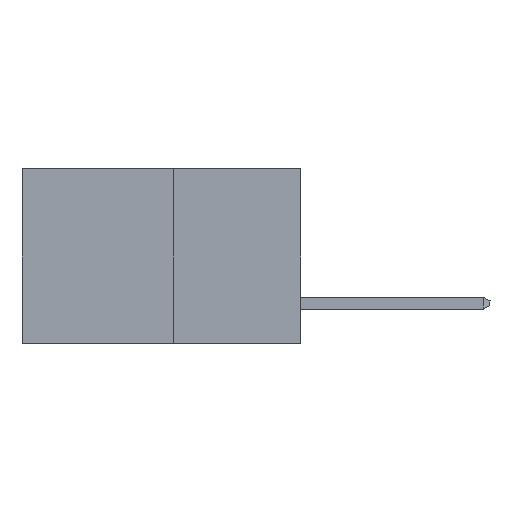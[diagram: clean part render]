
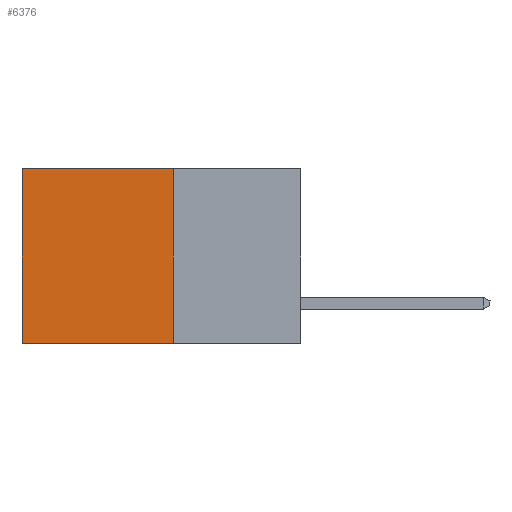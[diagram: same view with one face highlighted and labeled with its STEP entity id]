
A CAD part, left-side view. The second image highlights one B-rep face of the part: STEP entity #6376.
In plain terms, the highlighted planar face has unit normal (-1, 0, 0).
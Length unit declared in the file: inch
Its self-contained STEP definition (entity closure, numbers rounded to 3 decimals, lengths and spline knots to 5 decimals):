
#24 = EDGE_CURVE ( 'NONE', #12196, #17083, #17181, .T. ) ;
#222 = VERTEX_POINT ( 'NONE', #9934 ) ;
#316 = LINE ( 'NONE', #12168, #14150 ) ;
#854 = CARTESIAN_POINT ( 'NONE',  ( 0.277, 0.59, 0. ) ) ;
#1708 = EDGE_LOOP ( 'NONE', ( #17193, #6873, #13920, #2219 ) ) ;
#2219 = ORIENTED_EDGE ( 'NONE', *, *, #24, .T. ) ;
#3734 = DIRECTION ( 'NONE',  ( 1., 0., 0. ) ) ;
#3735 = AXIS2_PLACEMENT_3D ( 'NONE', #12021, #3734, #13391 ) ;
#4505 = VERTEX_POINT ( 'NONE', #7447 ) ;
#5271 = VECTOR ( 'NONE', #15471, 39.37008 ) ;
#5319 = DIRECTION ( 'NONE',  ( 0., 0., -1. ) ) ;
#5929 = CARTESIAN_POINT ( 'NONE',  ( 0.277, 0.27, -0.37 ) ) ;
#6088 = EDGE_CURVE ( 'NONE', #12196, #4505, #12887, .T. ) ;
#6343 = CARTESIAN_POINT ( 'NONE',  ( 0.277, 0.27, 0. ) ) ;
#6376 = ADVANCED_FACE ( 'NONE', ( #12042 ), #6541, .F. ) ;
#6541 = PLANE ( 'NONE',  #3735 ) ;
#6873 = ORIENTED_EDGE ( 'NONE', *, *, #12898, .F. ) ;
#7422 = CARTESIAN_POINT ( 'NONE',  ( 0.277, 0.27, -0.37 ) ) ;
#7447 = CARTESIAN_POINT ( 'NONE',  ( 0.277, 0.27, -0.37 ) ) ;
#9418 = LINE ( 'NONE', #5929, #5271 ) ;
#9934 = CARTESIAN_POINT ( 'NONE',  ( 0.277, 0.59, -0.37 ) ) ;
#10205 = VECTOR ( 'NONE', #12155, 39.37008 ) ;
#10402 = EDGE_CURVE ( 'NONE', #17083, #222, #316, .T. ) ;
#12021 = CARTESIAN_POINT ( 'NONE',  ( 0.277, 0.27, -0.37 ) ) ;
#12042 = FACE_OUTER_BOUND ( 'NONE', #1708, .T. ) ;
#12155 = DIRECTION ( 'NONE',  ( 0., 1., 0. ) ) ;
#12168 = CARTESIAN_POINT ( 'NONE',  ( 0.277, 0.59, -0.37 ) ) ;
#12196 = VERTEX_POINT ( 'NONE', #14121 ) ;
#12887 = LINE ( 'NONE', #7422, #16733 ) ;
#12898 = EDGE_CURVE ( 'NONE', #4505, #222, #9418, .T. ) ;
#13391 = DIRECTION ( 'NONE',  ( 0., 0., -1. ) ) ;
#13920 = ORIENTED_EDGE ( 'NONE', *, *, #6088, .F. ) ;
#14121 = CARTESIAN_POINT ( 'NONE',  ( 0.277, 0.27, 0. ) ) ;
#14150 = VECTOR ( 'NONE', #5319, 39.37008 ) ;
#15471 = DIRECTION ( 'NONE',  ( 0., 1., 0. ) ) ;
#16725 = DIRECTION ( 'NONE',  ( 0., 0., -1. ) ) ;
#16733 = VECTOR ( 'NONE', #16725, 39.37008 ) ;
#17083 = VERTEX_POINT ( 'NONE', #854 ) ;
#17181 = LINE ( 'NONE', #6343, #10205 ) ;
#17193 = ORIENTED_EDGE ( 'NONE', *, *, #10402, .T. ) ;
